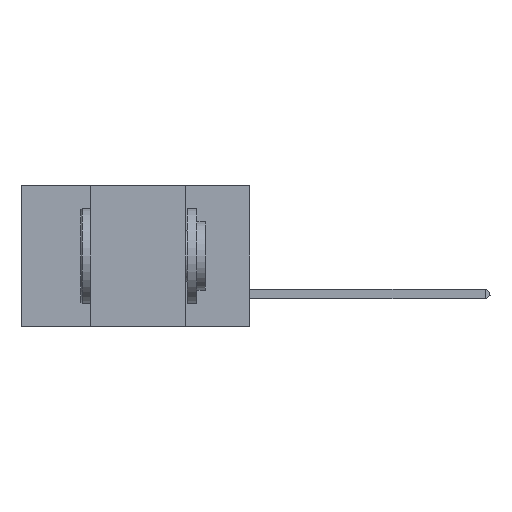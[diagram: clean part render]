
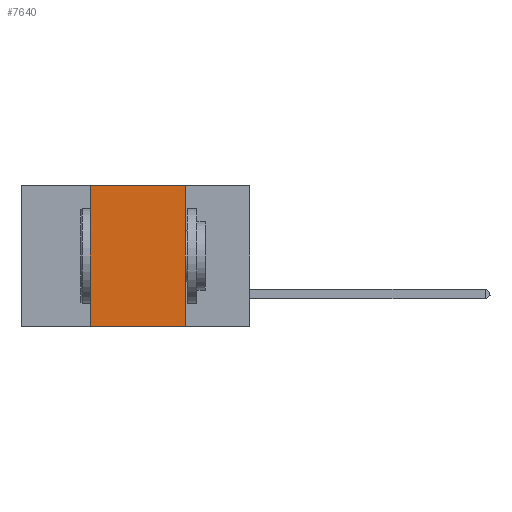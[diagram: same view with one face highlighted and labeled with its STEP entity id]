
A CAD part, left-side view. The second image highlights one B-rep face of the part: STEP entity #7640.
In plain terms, the highlighted planar face has unit normal (-1, 0, 0).
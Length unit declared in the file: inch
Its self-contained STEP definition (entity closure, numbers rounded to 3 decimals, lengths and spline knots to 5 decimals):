
#71 = VECTOR ( 'NONE', #9424, 39.37008 ) ;
#304 = DIRECTION ( 'NONE',  ( 1., 0., 0. ) ) ;
#2041 = VECTOR ( 'NONE', #3214, 39.37008 ) ;
#2456 = CARTESIAN_POINT ( 'NONE',  ( 0., 0.17, -0.37 ) ) ;
#2810 = AXIS2_PLACEMENT_3D ( 'NONE', #17195, #304, #15594 ) ;
#3102 = CARTESIAN_POINT ( 'NONE',  ( 0., 0.42, 0. ) ) ;
#3214 = DIRECTION ( 'NONE',  ( 0., -1., 0. ) ) ;
#3753 = CARTESIAN_POINT ( 'NONE',  ( 0., 0.17, 0. ) ) ;
#4690 = DIRECTION ( 'NONE',  ( 0., 0., 1. ) ) ;
#6190 = LINE ( 'NONE', #17787, #71 ) ;
#6745 = VERTEX_POINT ( 'NONE', #13257 ) ;
#7640 = ADVANCED_FACE ( 'NONE', ( #18713 ), #10523, .F. ) ;
#7724 = EDGE_CURVE ( 'NONE', #14554, #13812, #13169, .T. ) ;
#9204 = EDGE_CURVE ( 'NONE', #14554, #11974, #21284, .T. ) ;
#9424 = DIRECTION ( 'NONE',  ( 0., -1., 0. ) ) ;
#10523 = PLANE ( 'NONE',  #2810 ) ;
#10766 = LINE ( 'NONE', #3753, #14492 ) ;
#11935 = EDGE_CURVE ( 'NONE', #11974, #6745, #6190, .T. ) ;
#11974 = VERTEX_POINT ( 'NONE', #3102 ) ;
#11995 = ORIENTED_EDGE ( 'NONE', *, *, #16231, .F. ) ;
#12999 = ORIENTED_EDGE ( 'NONE', *, *, #11935, .F. ) ;
#13169 = LINE ( 'NONE', #15034, #2041 ) ;
#13257 = CARTESIAN_POINT ( 'NONE',  ( 0., 0.17, 0. ) ) ;
#13812 = VERTEX_POINT ( 'NONE', #2456 ) ;
#14056 = CARTESIAN_POINT ( 'NONE',  ( 0., 0.42, -0.37 ) ) ;
#14492 = VECTOR ( 'NONE', #15904, 39.37008 ) ;
#14554 = VERTEX_POINT ( 'NONE', #14056 ) ;
#15034 = CARTESIAN_POINT ( 'NONE',  ( 0., 0.6, -0.37 ) ) ;
#15594 = DIRECTION ( 'NONE',  ( 0., 0., -1. ) ) ;
#15904 = DIRECTION ( 'NONE',  ( 0., 0., -1. ) ) ;
#16231 = EDGE_CURVE ( 'NONE', #6745, #13812, #10766, .T. ) ;
#16802 = ORIENTED_EDGE ( 'NONE', *, *, #9204, .F. ) ;
#16842 = VECTOR ( 'NONE', #4690, 39.37008 ) ;
#17195 = CARTESIAN_POINT ( 'NONE',  ( 0., 0.6, 0. ) ) ;
#17787 = CARTESIAN_POINT ( 'NONE',  ( 0., 0.6, 0. ) ) ;
#18713 = FACE_OUTER_BOUND ( 'NONE', #20355, .T. ) ;
#20283 = CARTESIAN_POINT ( 'NONE',  ( 0., 0.42, 0. ) ) ;
#20355 = EDGE_LOOP ( 'NONE', ( #11995, #12999, #16802, #20394 ) ) ;
#20394 = ORIENTED_EDGE ( 'NONE', *, *, #7724, .T. ) ;
#21284 = LINE ( 'NONE', #20283, #16842 ) ;
